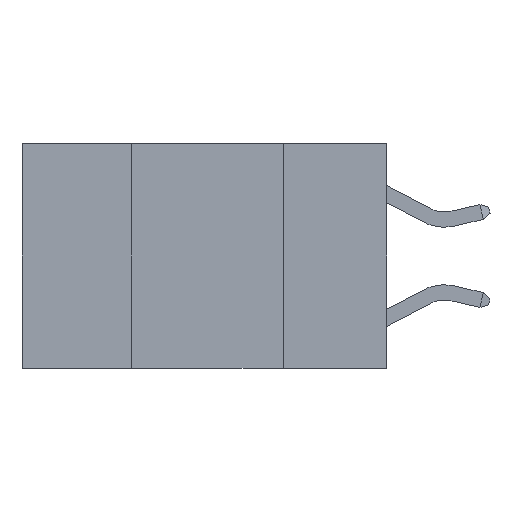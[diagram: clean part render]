
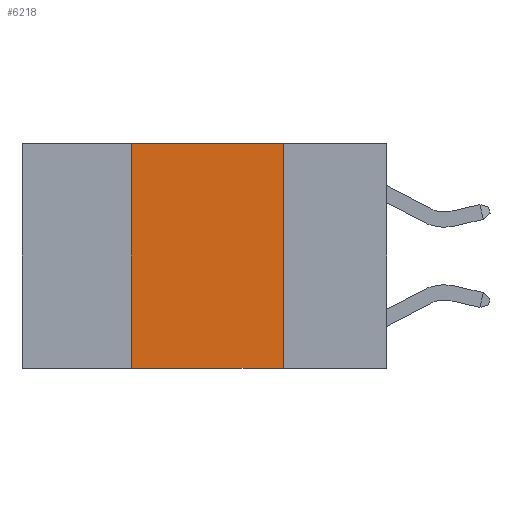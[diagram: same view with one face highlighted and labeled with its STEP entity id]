
A CAD part, left-side view. The second image highlights one B-rep face of the part: STEP entity #6218.
In plain terms, the highlighted planar face has unit normal (-1, 0, 0).
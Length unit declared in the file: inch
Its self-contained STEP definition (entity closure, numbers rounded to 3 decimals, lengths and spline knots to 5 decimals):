
#838 = CARTESIAN_POINT ( 'NONE',  ( 0., 0.42, 0. ) ) ;
#1808 = VECTOR ( 'NONE', #11102, 39.37008 ) ;
#1963 = CARTESIAN_POINT ( 'NONE',  ( 0., 0.6, 0. ) ) ;
#2249 = CARTESIAN_POINT ( 'NONE',  ( 0., 0.17, 0. ) ) ;
#3418 = ORIENTED_EDGE ( 'NONE', *, *, #8331, .T. ) ;
#4264 = VECTOR ( 'NONE', #8333, 39.37008 ) ;
#4285 = EDGE_CURVE ( 'NONE', #7941, #22141, #18409, .T. ) ;
#4661 = VERTEX_POINT ( 'NONE', #12485 ) ;
#5424 = VERTEX_POINT ( 'NONE', #21839 ) ;
#6102 = EDGE_LOOP ( 'NONE', ( #7310, #17224, #12906, #3418 ) ) ;
#6218 = ADVANCED_FACE ( 'NONE', ( #15504 ), #17463, .F. ) ;
#7310 = ORIENTED_EDGE ( 'NONE', *, *, #11671, .F. ) ;
#7941 = VERTEX_POINT ( 'NONE', #16482 ) ;
#8331 = EDGE_CURVE ( 'NONE', #5424, #4661, #14289, .T. ) ;
#8333 = DIRECTION ( 'NONE',  ( 0., -1., 0. ) ) ;
#10046 = CARTESIAN_POINT ( 'NONE',  ( 0., 0.6, 0. ) ) ;
#11102 = DIRECTION ( 'NONE',  ( 0., 0., -1. ) ) ;
#11671 = EDGE_CURVE ( 'NONE', #22141, #4661, #18008, .T. ) ;
#11938 = DIRECTION ( 'NONE',  ( 0., 0., -1. ) ) ;
#12318 = VECTOR ( 'NONE', #21534, 39.37008 ) ;
#12485 = CARTESIAN_POINT ( 'NONE',  ( 0., 0.17, -0.37 ) ) ;
#12906 = ORIENTED_EDGE ( 'NONE', *, *, #16034, .F. ) ;
#12916 = LINE ( 'NONE', #838, #12318 ) ;
#13883 = CARTESIAN_POINT ( 'NONE',  ( 0., 0.6, -0.37 ) ) ;
#14289 = LINE ( 'NONE', #13883, #4264 ) ;
#15504 = FACE_OUTER_BOUND ( 'NONE', #6102, .T. ) ;
#16034 = EDGE_CURVE ( 'NONE', #5424, #7941, #12916, .T. ) ;
#16482 = CARTESIAN_POINT ( 'NONE',  ( 0., 0.42, 0. ) ) ;
#17015 = DIRECTION ( 'NONE',  ( 0., -1., 0. ) ) ;
#17224 = ORIENTED_EDGE ( 'NONE', *, *, #4285, .F. ) ;
#17463 = PLANE ( 'NONE',  #23176 ) ;
#18008 = LINE ( 'NONE', #18483, #1808 ) ;
#18409 = LINE ( 'NONE', #1963, #23367 ) ;
#18483 = CARTESIAN_POINT ( 'NONE',  ( 0., 0.17, 0. ) ) ;
#21534 = DIRECTION ( 'NONE',  ( 0., 0., 1. ) ) ;
#21839 = CARTESIAN_POINT ( 'NONE',  ( 0., 0.42, -0.37 ) ) ;
#22141 = VERTEX_POINT ( 'NONE', #2249 ) ;
#23058 = DIRECTION ( 'NONE',  ( 1., 0., 0. ) ) ;
#23176 = AXIS2_PLACEMENT_3D ( 'NONE', #10046, #23058, #11938 ) ;
#23367 = VECTOR ( 'NONE', #17015, 39.37008 ) ;
